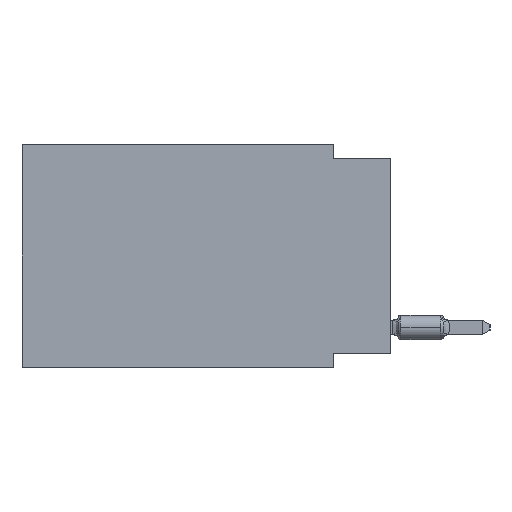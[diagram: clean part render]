
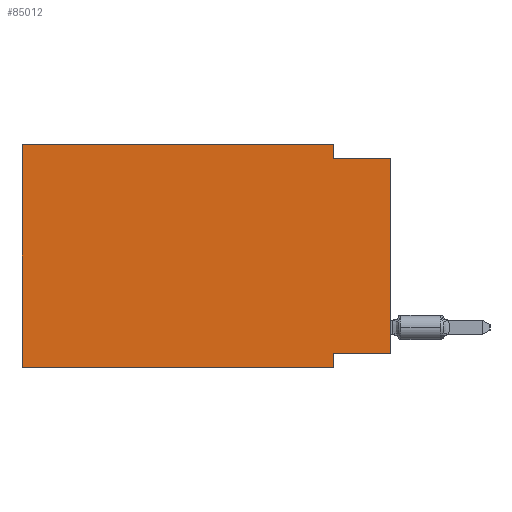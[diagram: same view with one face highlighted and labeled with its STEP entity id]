
A CAD part, left-side view. The second image highlights one B-rep face of the part: STEP entity #85012.
In plain terms, the highlighted planar face has unit normal (-1, 0, 0).
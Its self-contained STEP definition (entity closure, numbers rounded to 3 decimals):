
#1350 = LINE ( 'NONE', #82915, #59661 ) ;
#2226 = FACE_OUTER_BOUND ( 'NONE', #84784, .T. ) ;
#2356 = VECTOR ( 'NONE', #83768, 1000. ) ;
#2664 = CARTESIAN_POINT ( 'NONE',  ( 0., 16.383, 0. ) ) ;
#3063 = LINE ( 'NONE', #15783, #2356 ) ;
#3802 = AXIS2_PLACEMENT_3D ( 'NONE', #2664, #50428, #10080 ) ;
#6040 = VERTEX_POINT ( 'NONE', #76361 ) ;
#6176 = EDGE_CURVE ( 'NONE', #15257, #46447, #58288, .T. ) ;
#8648 = CARTESIAN_POINT ( 'NONE',  ( 0., 2.54, -9.271 ) ) ;
#10080 = DIRECTION ( 'NONE',  ( 0., 0., -1. ) ) ;
#10128 = LINE ( 'NONE', #85559, #12971 ) ;
#10676 = LINE ( 'NONE', #65075, #61771 ) ;
#10769 = LINE ( 'NONE', #50688, #47126 ) ;
#12214 = EDGE_CURVE ( 'NONE', #15257, #23511, #65782, .T. ) ;
#12971 = VECTOR ( 'NONE', #32016, 1000. ) ;
#14041 = VECTOR ( 'NONE', #80151, 1000. ) ;
#14523 = CARTESIAN_POINT ( 'NONE',  ( 0., 2.54, 0. ) ) ;
#15257 = VERTEX_POINT ( 'NONE', #72704 ) ;
#15783 = CARTESIAN_POINT ( 'NONE',  ( 0., 16.383, 0. ) ) ;
#16046 = ORIENTED_EDGE ( 'NONE', *, *, #53776, .F. ) ;
#17259 = DIRECTION ( 'NONE',  ( 0., 0., -1. ) ) ;
#17329 = ORIENTED_EDGE ( 'NONE', *, *, #18657, .F. ) ;
#18378 = DIRECTION ( 'NONE',  ( 0., 0., 1. ) ) ;
#18657 = EDGE_CURVE ( 'NONE', #46447, #19710, #3063, .T. ) ;
#19710 = VERTEX_POINT ( 'NONE', #14523 ) ;
#23511 = VERTEX_POINT ( 'NONE', #73334 ) ;
#24525 = CARTESIAN_POINT ( 'NONE',  ( 0., 16.383, 0. ) ) ;
#32016 = DIRECTION ( 'NONE',  ( 0., 0., -1. ) ) ;
#35015 = ORIENTED_EDGE ( 'NONE', *, *, #6176, .F. ) ;
#39250 = ORIENTED_EDGE ( 'NONE', *, *, #70463, .F. ) ;
#41397 = VECTOR ( 'NONE', #18378, 1000. ) ;
#41947 = CARTESIAN_POINT ( 'NONE',  ( 0., 2.54, -0.635 ) ) ;
#43102 = VERTEX_POINT ( 'NONE', #8648 ) ;
#43413 = PLANE ( 'NONE',  #3802 ) ;
#44102 = DIRECTION ( 'NONE',  ( 0., 0., 1. ) ) ;
#44965 = CARTESIAN_POINT ( 'NONE',  ( 0., 0., -0.635 ) ) ;
#45044 = ORIENTED_EDGE ( 'NONE', *, *, #47378, .T. ) ;
#45573 = DIRECTION ( 'NONE',  ( 0., -1., 0. ) ) ;
#46447 = VERTEX_POINT ( 'NONE', #55325 ) ;
#47126 = VECTOR ( 'NONE', #44102, 1000. ) ;
#47378 = EDGE_CURVE ( 'NONE', #6040, #58629, #10769, .T. ) ;
#49156 = ORIENTED_EDGE ( 'NONE', *, *, #51085, .F. ) ;
#50428 = DIRECTION ( 'NONE',  ( 1., 0., 0. ) ) ;
#50688 = CARTESIAN_POINT ( 'NONE',  ( 0., 0., 0. ) ) ;
#51085 = EDGE_CURVE ( 'NONE', #19710, #62330, #10676, .T. ) ;
#53776 = EDGE_CURVE ( 'NONE', #43102, #23511, #10128, .T. ) ;
#55325 = CARTESIAN_POINT ( 'NONE',  ( 0., 16.383, 0. ) ) ;
#55695 = DIRECTION ( 'NONE',  ( 0., 1., 0. ) ) ;
#57037 = ORIENTED_EDGE ( 'NONE', *, *, #81683, .F. ) ;
#58288 = LINE ( 'NONE', #24525, #41397 ) ;
#58629 = VERTEX_POINT ( 'NONE', #44965 ) ;
#59661 = VECTOR ( 'NONE', #55695, 1000. ) ;
#60059 = CARTESIAN_POINT ( 'NONE',  ( 0., 16.383, -9.906 ) ) ;
#61771 = VECTOR ( 'NONE', #17259, 1000. ) ;
#62330 = VERTEX_POINT ( 'NONE', #41947 ) ;
#65075 = CARTESIAN_POINT ( 'NONE',  ( 0., 2.54, 0. ) ) ;
#65668 = LINE ( 'NONE', #73128, #14041 ) ;
#65782 = LINE ( 'NONE', #60059, #80138 ) ;
#70463 = EDGE_CURVE ( 'NONE', #62330, #58629, #65668, .T. ) ;
#72704 = CARTESIAN_POINT ( 'NONE',  ( 0., 16.383, -9.906 ) ) ;
#73128 = CARTESIAN_POINT ( 'NONE',  ( 0., 0., -0.635 ) ) ;
#73334 = CARTESIAN_POINT ( 'NONE',  ( 0., 2.54, -9.906 ) ) ;
#76361 = CARTESIAN_POINT ( 'NONE',  ( 0., 0., -9.271 ) ) ;
#80138 = VECTOR ( 'NONE', #45573, 1000. ) ;
#80151 = DIRECTION ( 'NONE',  ( 0., -1., 0. ) ) ;
#81683 = EDGE_CURVE ( 'NONE', #6040, #43102, #1350, .T. ) ;
#82915 = CARTESIAN_POINT ( 'NONE',  ( 0., 0., -9.271 ) ) ;
#83768 = DIRECTION ( 'NONE',  ( 0., -1., 0. ) ) ;
#84480 = ORIENTED_EDGE ( 'NONE', *, *, #12214, .T. ) ;
#84784 = EDGE_LOOP ( 'NONE', ( #45044, #39250, #49156, #17329, #35015, #84480, #16046, #57037 ) ) ;
#85012 = ADVANCED_FACE ( 'NONE', ( #2226 ), #43413, .F. ) ;
#85559 = CARTESIAN_POINT ( 'NONE',  ( 0., 2.54, -9.906 ) ) ;
